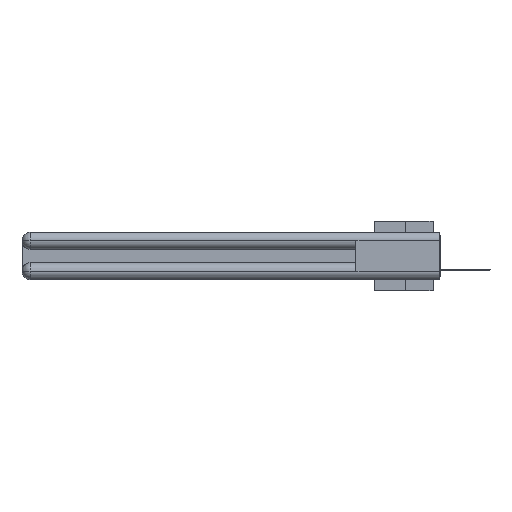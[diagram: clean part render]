
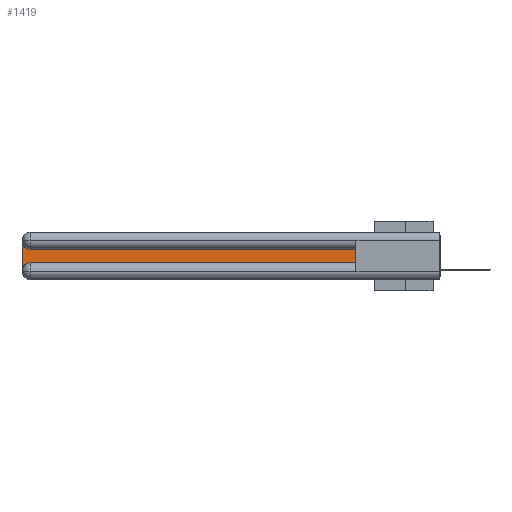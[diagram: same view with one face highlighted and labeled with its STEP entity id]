
A CAD part, left-side view. The second image highlights one B-rep face of the part: STEP entity #1419.
In plain terms, the highlighted planar face has unit normal (-1, 0, 0).
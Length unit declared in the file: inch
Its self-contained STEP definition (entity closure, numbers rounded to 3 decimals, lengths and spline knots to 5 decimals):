
#1366 = DIRECTION ( 'NONE',  ( 0., 0., -1. ) ) ;
#1419 = ADVANCED_FACE ( 'NONE', ( #6353 ), #24767, .F. ) ;
#2636 = DIRECTION ( 'NONE',  ( 1., 0., 0. ) ) ;
#3546 = DIRECTION ( 'NONE',  ( 1., 0., 0. ) ) ;
#4297 = CARTESIAN_POINT ( 'NONE',  ( 0.075, 2.94, -0.1225 ) ) ;
#4529 = LINE ( 'NONE', #8053, #7803 ) ;
#4765 = VERTEX_POINT ( 'NONE', #15230 ) ;
#4878 = CIRCLE ( 'NONE', #26045, 0.06 ) ;
#5418 = CARTESIAN_POINT ( 'NONE',  ( 0.075, 2.94, -0.2775 ) ) ;
#5563 = CARTESIAN_POINT ( 'NONE',  ( 0.075, 0.6, -0.2175 ) ) ;
#6353 = FACE_OUTER_BOUND ( 'NONE', #26674, .T. ) ;
#6524 = CARTESIAN_POINT ( 'NONE',  ( 0.075, 0.6, -0.2175 ) ) ;
#6785 = VERTEX_POINT ( 'NONE', #4297 ) ;
#7091 = VERTEX_POINT ( 'NONE', #24076 ) ;
#7145 = LINE ( 'NONE', #5563, #28927 ) ;
#7148 = EDGE_CURVE ( 'NONE', #4765, #6785, #4529, .T. ) ;
#7803 = VECTOR ( 'NONE', #24377, 39.37008 ) ;
#7870 = ORIENTED_EDGE ( 'NONE', *, *, #24193, .T. ) ;
#8053 = CARTESIAN_POINT ( 'NONE',  ( 0.075, 0.6, -0.1225 ) ) ;
#8222 = DIRECTION ( 'NONE',  ( 0., 0., 1. ) ) ;
#9097 = CARTESIAN_POINT ( 'NONE',  ( 0.075, 3., -0.0625 ) ) ;
#10021 = ORIENTED_EDGE ( 'NONE', *, *, #16870, .T. ) ;
#10083 = VERTEX_POINT ( 'NONE', #21790 ) ;
#11739 = AXIS2_PLACEMENT_3D ( 'NONE', #5418, #2636, #26380 ) ;
#11971 = VECTOR ( 'NONE', #23326, 39.37008 ) ;
#12967 = DIRECTION ( 'NONE',  ( 0., 0., -1. ) ) ;
#13313 = ORIENTED_EDGE ( 'NONE', *, *, #13972, .T. ) ;
#13972 = EDGE_CURVE ( 'NONE', #10083, #4765, #7145, .T. ) ;
#15230 = CARTESIAN_POINT ( 'NONE',  ( 0.075, 0.6, -0.1225 ) ) ;
#15735 = VECTOR ( 'NONE', #23041, 39.37008 ) ;
#16870 = EDGE_CURVE ( 'NONE', #18875, #10083, #18691, .T. ) ;
#17504 = EDGE_CURVE ( 'NONE', #25448, #7091, #26763, .T. ) ;
#18625 = AXIS2_PLACEMENT_3D ( 'NONE', #22070, #27142, #12967 ) ;
#18691 = LINE ( 'NONE', #6524, #15735 ) ;
#18875 = VERTEX_POINT ( 'NONE', #21405 ) ;
#21405 = CARTESIAN_POINT ( 'NONE',  ( 0.075, 2.94, -0.2175 ) ) ;
#21790 = CARTESIAN_POINT ( 'NONE',  ( 0.075, 0.6, -0.2175 ) ) ;
#22070 = CARTESIAN_POINT ( 'NONE',  ( 0.075, 3., -0.1225 ) ) ;
#22214 = ORIENTED_EDGE ( 'NONE', *, *, #28542, .T. ) ;
#22549 = ORIENTED_EDGE ( 'NONE', *, *, #7148, .T. ) ;
#23041 = DIRECTION ( 'NONE',  ( 0., -1., 0. ) ) ;
#23326 = DIRECTION ( 'NONE',  ( 0., 0., -1. ) ) ;
#24076 = CARTESIAN_POINT ( 'NONE',  ( 0.075, 3., -0.2775 ) ) ;
#24193 = EDGE_CURVE ( 'NONE', #7091, #18875, #27044, .T. ) ;
#24377 = DIRECTION ( 'NONE',  ( 0., 1., 0. ) ) ;
#24703 = CARTESIAN_POINT ( 'NONE',  ( 0.075, 2.94, -0.0625 ) ) ;
#24767 = PLANE ( 'NONE',  #18625 ) ;
#25448 = VERTEX_POINT ( 'NONE', #9097 ) ;
#26045 = AXIS2_PLACEMENT_3D ( 'NONE', #24703, #3546, #1366 ) ;
#26380 = DIRECTION ( 'NONE',  ( 0., 0., -1. ) ) ;
#26674 = EDGE_LOOP ( 'NONE', ( #22549, #22214, #27872, #7870, #10021, #13313 ) ) ;
#26763 = LINE ( 'NONE', #30418, #11971 ) ;
#27044 = CIRCLE ( 'NONE', #11739, 0.06 ) ;
#27142 = DIRECTION ( 'NONE',  ( 1., 0., 0. ) ) ;
#27872 = ORIENTED_EDGE ( 'NONE', *, *, #17504, .T. ) ;
#28542 = EDGE_CURVE ( 'NONE', #6785, #25448, #4878, .T. ) ;
#28927 = VECTOR ( 'NONE', #8222, 39.37008 ) ;
#30418 = CARTESIAN_POINT ( 'NONE',  ( 0.075, 3., -0.2175 ) ) ;
